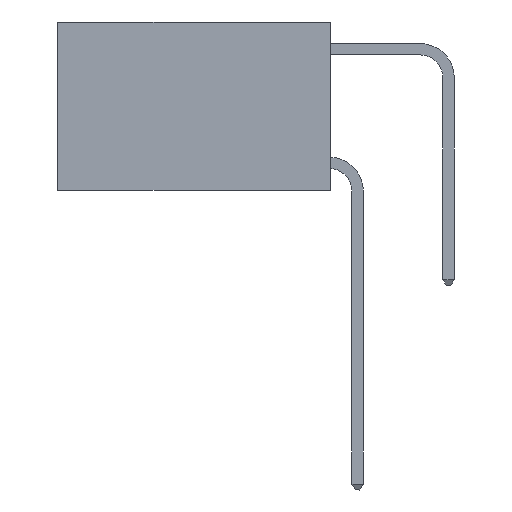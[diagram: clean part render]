
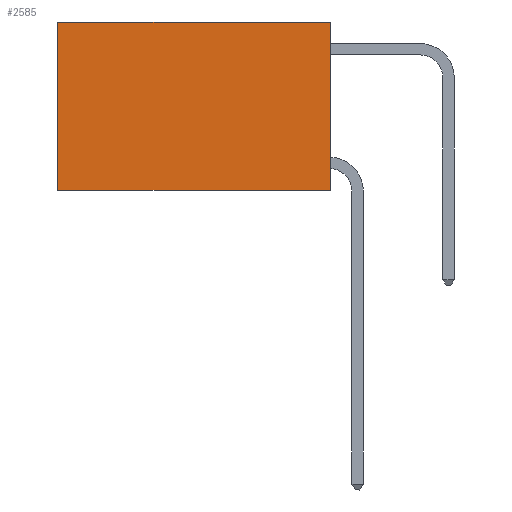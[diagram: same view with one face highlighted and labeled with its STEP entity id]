
A CAD part, left-side view. The second image highlights one B-rep face of the part: STEP entity #2585.
In plain terms, the highlighted planar face has unit normal (-1, 0, 0).
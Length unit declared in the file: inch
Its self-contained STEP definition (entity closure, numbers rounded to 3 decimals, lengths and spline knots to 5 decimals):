
#19 = VERTEX_POINT ( 'NONE', #12405 ) ;
#278 = DIRECTION ( 'NONE',  ( 1., 0., 0. ) ) ;
#586 = DIRECTION ( 'NONE',  ( 0., 1., 0. ) ) ;
#720 = FACE_OUTER_BOUND ( 'NONE', #5421, .T. ) ;
#1235 = LINE ( 'NONE', #5268, #11967 ) ;
#1437 = CARTESIAN_POINT ( 'NONE',  ( 0.2625, 0., 0. ) ) ;
#1850 = CARTESIAN_POINT ( 'NONE',  ( 0.2625, 0., 0. ) ) ;
#2083 = CARTESIAN_POINT ( 'NONE',  ( 0.2625, 0., -0.37 ) ) ;
#2484 = PLANE ( 'NONE',  #10872 ) ;
#2585 = ADVANCED_FACE ( 'NONE', ( #720 ), #2484, .F. ) ;
#2745 = EDGE_CURVE ( 'NONE', #9103, #19, #6701, .T. ) ;
#3247 = EDGE_CURVE ( 'NONE', #9103, #5465, #5064, .T. ) ;
#4209 = ORIENTED_EDGE ( 'NONE', *, *, #2745, .T. ) ;
#4608 = ORIENTED_EDGE ( 'NONE', *, *, #3247, .F. ) ;
#5064 = LINE ( 'NONE', #8999, #9625 ) ;
#5268 = CARTESIAN_POINT ( 'NONE',  ( 0.2625, 0.6, 0. ) ) ;
#5421 = EDGE_LOOP ( 'NONE', ( #7323, #11546, #4608, #4209 ) ) ;
#5465 = VERTEX_POINT ( 'NONE', #2083 ) ;
#6701 = LINE ( 'NONE', #1850, #9182 ) ;
#7167 = CARTESIAN_POINT ( 'NONE',  ( 0.2625, 0., 0. ) ) ;
#7323 = ORIENTED_EDGE ( 'NONE', *, *, #11558, .T. ) ;
#8013 = DIRECTION ( 'NONE',  ( 0., 1., 0. ) ) ;
#8579 = VERTEX_POINT ( 'NONE', #11500 ) ;
#8999 = CARTESIAN_POINT ( 'NONE',  ( 0.2625, 0., 0. ) ) ;
#9030 = LINE ( 'NONE', #12044, #12543 ) ;
#9103 = VERTEX_POINT ( 'NONE', #1437 ) ;
#9182 = VECTOR ( 'NONE', #586, 39.37008 ) ;
#9625 = VECTOR ( 'NONE', #11042, 39.37008 ) ;
#9835 = EDGE_CURVE ( 'NONE', #5465, #8579, #9030, .T. ) ;
#10872 = AXIS2_PLACEMENT_3D ( 'NONE', #7167, #278, #11129 ) ;
#11042 = DIRECTION ( 'NONE',  ( 0., 0., -1. ) ) ;
#11129 = DIRECTION ( 'NONE',  ( 0., 0., -1. ) ) ;
#11500 = CARTESIAN_POINT ( 'NONE',  ( 0.2625, 0.6, -0.37 ) ) ;
#11546 = ORIENTED_EDGE ( 'NONE', *, *, #9835, .F. ) ;
#11558 = EDGE_CURVE ( 'NONE', #19, #8579, #1235, .T. ) ;
#11967 = VECTOR ( 'NONE', #12199, 39.37008 ) ;
#12044 = CARTESIAN_POINT ( 'NONE',  ( 0.2625, 0., -0.37 ) ) ;
#12199 = DIRECTION ( 'NONE',  ( 0., 0., -1. ) ) ;
#12405 = CARTESIAN_POINT ( 'NONE',  ( 0.2625, 0.6, 0. ) ) ;
#12543 = VECTOR ( 'NONE', #8013, 39.37008 ) ;
